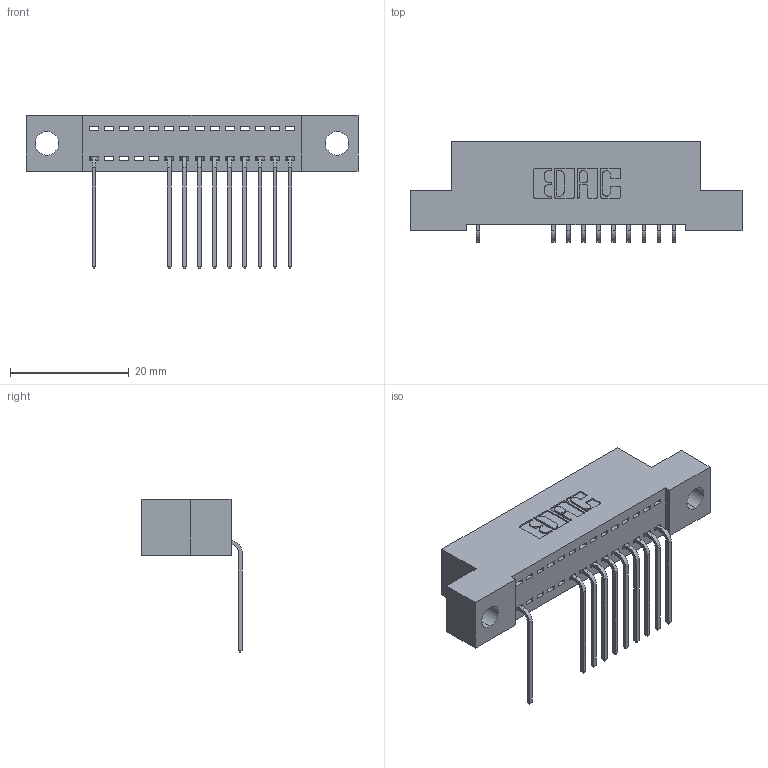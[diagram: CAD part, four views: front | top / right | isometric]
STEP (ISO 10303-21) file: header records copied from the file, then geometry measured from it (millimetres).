
FILE_DESCRIPTION (( 'STEP AP203' ), '1' );
FILE_NAME ('392-014-559-104.STEP', '2018-08-15T00:32:19', ( '' ), ( '' ), 'SwSTEP 2.0', 'SolidWorks 2016', '' );
FILE_SCHEMA (( 'CONFIG_CONTROL_DESIGN' ));
Length unit declared in the file: inch
Products named in the file (3): 342 Part_.156 TH; 345-292-001_558 559 Tail - 1; 392-014-559-104
Assembly tree (11 placements, depth 2):
  392-014-559-104
    342 Part_.156 TH
    345-292-001_558 559 Tail - 1  x10
Bounding box: 55.88 x 16.83 x 25.78 mm (x, y, z)
Volume: 4697 mm3; surface area: 6145.4 mm2
Topology: 11 solids, 11 shells, 758 faces, 2287 edges, 1510 vertices
Faces by surface type: plane 554, cylinder 204
Entity records: 12007 total; most frequent: CARTESIAN_POINT 2100, ORIENTED_EDGE 2054, DIRECTION 1823, EDGE_CURVE 1027, LINE 899, VECTOR 899, VERTEX_POINT 682, AXIS2_PLACEMENT_3D 462
